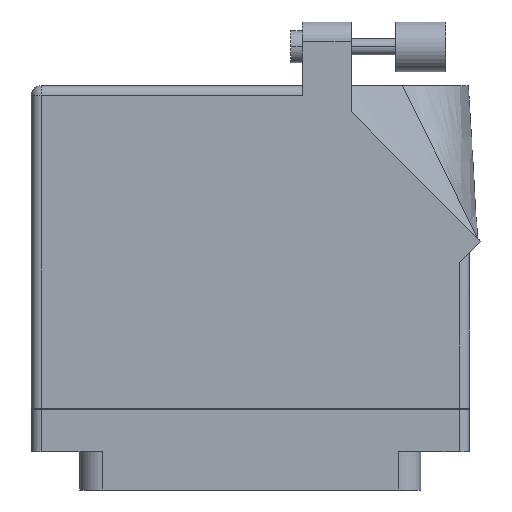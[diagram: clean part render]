
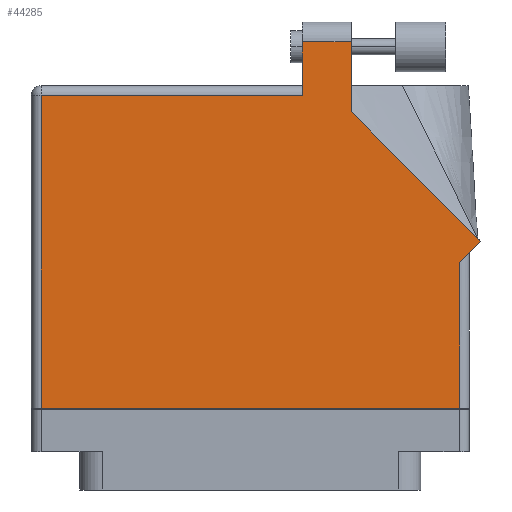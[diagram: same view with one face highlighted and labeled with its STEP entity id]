
A CAD part, front view. The second image highlights one B-rep face of the part: STEP entity #44285.
In plain terms, the highlighted face is planar.
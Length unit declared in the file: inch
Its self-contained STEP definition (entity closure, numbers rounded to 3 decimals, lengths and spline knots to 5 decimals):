
#2042 = ORIENTED_EDGE ( 'NONE', *, *, #66978, .T. ) ;
#2048 = VERTEX_POINT ( 'NONE', #17741 ) ;
#6755 = DIRECTION ( 'NONE',  ( 1., 0., 0. ) ) ;
#9755 = VERTEX_POINT ( 'NONE', #76358 ) ;
#10695 = ORIENTED_EDGE ( 'NONE', *, *, #44035, .T. ) ;
#12030 = LINE ( 'NONE', #54192, #51042 ) ;
#12310 = EDGE_LOOP ( 'NONE', ( #46349, #30774, #15060, #2042, #10695, #64328, #80623, #19297, #82076 ) ) ;
#13504 = EDGE_CURVE ( 'NONE', #49754, #61776, #12030, .T. ) ;
#14370 = DIRECTION ( 'NONE',  ( -0.707, 0.707, 0. ) ) ;
#15060 = ORIENTED_EDGE ( 'NONE', *, *, #27092, .T. ) ;
#15354 = EDGE_CURVE ( 'NONE', #43674, #49754, #35481, .T. ) ;
#17741 = CARTESIAN_POINT ( 'NONE',  ( 0.3275, 2.205, 0.765 ) ) ;
#19297 = ORIENTED_EDGE ( 'NONE', *, *, #65857, .T. ) ;
#19710 = CARTESIAN_POINT ( 'NONE',  ( 0.6345, 2.205, 0.765 ) ) ;
#20878 = VERTEX_POINT ( 'NONE', #35365 ) ;
#21999 = DIRECTION ( 'NONE',  ( 0., 1., 0. ) ) ;
#25890 = CARTESIAN_POINT ( 'NONE',  ( -1.3775, 1.93, 0.765 ) ) ;
#26268 = LINE ( 'NONE', #57448, #45340 ) ;
#26408 = CARTESIAN_POINT ( 'NONE',  ( 0.3275, 1.93, 0.765 ) ) ;
#27092 = EDGE_CURVE ( 'NONE', #2048, #60844, #63305, .T. ) ;
#28322 = LINE ( 'NONE', #54019, #39312 ) ;
#29854 = EDGE_CURVE ( 'NONE', #41121, #9755, #26268, .T. ) ;
#29855 = DIRECTION ( 'NONE',  ( 0., 1., 0. ) ) ;
#30774 = ORIENTED_EDGE ( 'NONE', *, *, #51266, .T. ) ;
#34686 = DIRECTION ( 'NONE',  ( -1., 0., 0. ) ) ;
#35365 = CARTESIAN_POINT ( 'NONE',  ( -1.3155, 1.868, 0.765 ) ) ;
#35481 = LINE ( 'NONE', #72535, #50509 ) ;
#37091 = EDGE_CURVE ( 'NONE', #9755, #42578, #56608, .T. ) ;
#37930 = VECTOR ( 'NONE', #72552, 39.37008 ) ;
#38483 = CARTESIAN_POINT ( 'NONE',  ( -1.3155, -0.1, 0.765 ) ) ;
#39312 = VECTOR ( 'NONE', #34686, 39.37008 ) ;
#39562 = VECTOR ( 'NONE', #29855, 39.37008 ) ;
#40046 = VECTOR ( 'NONE', #68058, 39.37008 ) ;
#41121 = VERTEX_POINT ( 'NONE', #38483 ) ;
#41553 = CARTESIAN_POINT ( 'NONE',  ( 1.44821, 0.95071, 0.765 ) ) ;
#42244 = VECTOR ( 'NONE', #78582, 39.37008 ) ;
#42578 = VERTEX_POINT ( 'NONE', #44233 ) ;
#43674 = VERTEX_POINT ( 'NONE', #41553 ) ;
#44035 = EDGE_CURVE ( 'NONE', #20878, #41121, #61100, .T. ) ;
#44233 = CARTESIAN_POINT ( 'NONE',  ( 1.3155, 0.818, 0.765 ) ) ;
#44285 = ADVANCED_FACE ( 'NONE', ( #79905 ), #70826, .F. ) ;
#45340 = VECTOR ( 'NONE', #6755, 39.37008 ) ;
#46349 = ORIENTED_EDGE ( 'NONE', *, *, #13504, .T. ) ;
#46947 = CARTESIAN_POINT ( 'NONE',  ( 1.3775, 0.88, 0.765 ) ) ;
#49744 = LINE ( 'NONE', #51923, #59776 ) ;
#49754 = VERTEX_POINT ( 'NONE', #76244 ) ;
#50509 = VECTOR ( 'NONE', #14370, 39.37008 ) ;
#51042 = VECTOR ( 'NONE', #21999, 39.37008 ) ;
#51266 = EDGE_CURVE ( 'NONE', #61776, #2048, #28322, .T. ) ;
#51846 = AXIS2_PLACEMENT_3D ( 'NONE', #25890, #64997, #70556 ) ;
#51923 = CARTESIAN_POINT ( 'NONE',  ( -1.3775, 1.868, 0.765 ) ) ;
#54019 = CARTESIAN_POINT ( 'NONE',  ( 0.3275, 2.205, 0.765 ) ) ;
#54192 = CARTESIAN_POINT ( 'NONE',  ( 0.6345, 1.76442, 0.765 ) ) ;
#56424 = CARTESIAN_POINT ( 'NONE',  ( -1.3155, -0.1, 0.765 ) ) ;
#56608 = LINE ( 'NONE', #61251, #39562 ) ;
#57448 = CARTESIAN_POINT ( 'NONE',  ( -1.3775, -0.1, 0.765 ) ) ;
#58361 = DIRECTION ( 'NONE',  ( -1., 0., 0. ) ) ;
#59684 = CARTESIAN_POINT ( 'NONE',  ( 0.3275, 1.868, 0.765 ) ) ;
#59776 = VECTOR ( 'NONE', #58361, 39.37008 ) ;
#60844 = VERTEX_POINT ( 'NONE', #59684 ) ;
#61100 = LINE ( 'NONE', #56424, #40046 ) ;
#61251 = CARTESIAN_POINT ( 'NONE',  ( 1.3155, 0.88, 0.765 ) ) ;
#61776 = VERTEX_POINT ( 'NONE', #19710 ) ;
#63305 = LINE ( 'NONE', #26408, #42244 ) ;
#64328 = ORIENTED_EDGE ( 'NONE', *, *, #29854, .T. ) ;
#64929 = LINE ( 'NONE', #46947, #37930 ) ;
#64997 = DIRECTION ( 'NONE',  ( 0., 0., -1. ) ) ;
#65857 = EDGE_CURVE ( 'NONE', #42578, #43674, #64929, .T. ) ;
#66978 = EDGE_CURVE ( 'NONE', #60844, #20878, #49744, .T. ) ;
#68058 = DIRECTION ( 'NONE',  ( 0., -1., 0. ) ) ;
#70556 = DIRECTION ( 'NONE',  ( -1., 0., 0. ) ) ;
#70826 = PLANE ( 'NONE',  #51846 ) ;
#72535 = CARTESIAN_POINT ( 'NONE',  ( 1.44821, 0.95071, 0.765 ) ) ;
#72552 = DIRECTION ( 'NONE',  ( 0.707, 0.707, 0. ) ) ;
#76244 = CARTESIAN_POINT ( 'NONE',  ( 0.6345, 1.76442, 0.765 ) ) ;
#76358 = CARTESIAN_POINT ( 'NONE',  ( 1.3155, -0.1, 0.765 ) ) ;
#78582 = DIRECTION ( 'NONE',  ( 0., -1., 0. ) ) ;
#79905 = FACE_OUTER_BOUND ( 'NONE', #12310, .T. ) ;
#80623 = ORIENTED_EDGE ( 'NONE', *, *, #37091, .T. ) ;
#82076 = ORIENTED_EDGE ( 'NONE', *, *, #15354, .T. ) ;
